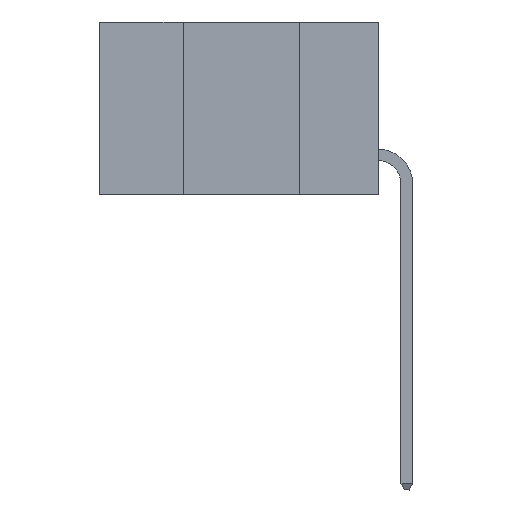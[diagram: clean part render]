
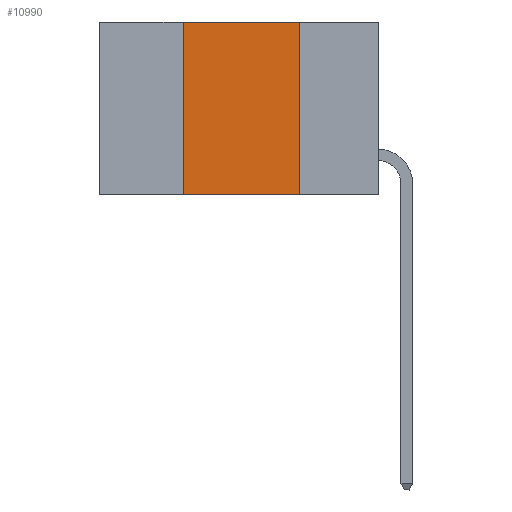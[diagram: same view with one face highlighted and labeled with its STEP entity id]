
A CAD part, left-side view. The second image highlights one B-rep face of the part: STEP entity #10990.
In plain terms, the highlighted planar face has unit normal (-1, 0, 0).
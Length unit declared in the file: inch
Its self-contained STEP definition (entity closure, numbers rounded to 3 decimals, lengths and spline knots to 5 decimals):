
#491 = EDGE_CURVE ( 'NONE', #5956, #13332, #5429, .T. ) ;
#874 = EDGE_LOOP ( 'NONE', ( #14414, #11052, #2569, #13044 ) ) ;
#1009 = DIRECTION ( 'NONE',  ( 0., 0., 1. ) ) ;
#1299 = DIRECTION ( 'NONE',  ( 0., -1., 0. ) ) ;
#2569 = ORIENTED_EDGE ( 'NONE', *, *, #491, .F. ) ;
#2683 = CARTESIAN_POINT ( 'NONE',  ( 0., 0.6, 0. ) ) ;
#2935 = VERTEX_POINT ( 'NONE', #14558 ) ;
#2951 = CARTESIAN_POINT ( 'NONE',  ( 0., 0.42, 0. ) ) ;
#3145 = EDGE_CURVE ( 'NONE', #2935, #16060, #17290, .T. ) ;
#4485 = PLANE ( 'NONE',  #13430 ) ;
#5429 = LINE ( 'NONE', #13811, #9124 ) ;
#5556 = LINE ( 'NONE', #15498, #8524 ) ;
#5648 = EDGE_CURVE ( 'NONE', #13332, #2935, #5556, .T. ) ;
#5956 = VERTEX_POINT ( 'NONE', #14962 ) ;
#7456 = CARTESIAN_POINT ( 'NONE',  ( 0., 0.17, -0.37 ) ) ;
#7720 = DIRECTION ( 'NONE',  ( 0., -1., 0. ) ) ;
#8524 = VECTOR ( 'NONE', #1299, 39.37008 ) ;
#8714 = FACE_OUTER_BOUND ( 'NONE', #874, .T. ) ;
#9124 = VECTOR ( 'NONE', #1009, 39.37008 ) ;
#9308 = VECTOR ( 'NONE', #7720, 39.37008 ) ;
#10055 = VECTOR ( 'NONE', #11528, 39.37008 ) ;
#10190 = LINE ( 'NONE', #11851, #9308 ) ;
#10990 = ADVANCED_FACE ( 'NONE', ( #8714 ), #4485, .F. ) ;
#11052 = ORIENTED_EDGE ( 'NONE', *, *, #5648, .F. ) ;
#11528 = DIRECTION ( 'NONE',  ( 0., 0., -1. ) ) ;
#11851 = CARTESIAN_POINT ( 'NONE',  ( 0., 0.6, -0.37 ) ) ;
#13044 = ORIENTED_EDGE ( 'NONE', *, *, #17074, .T. ) ;
#13332 = VERTEX_POINT ( 'NONE', #2951 ) ;
#13430 = AXIS2_PLACEMENT_3D ( 'NONE', #2683, #14338, #15842 ) ;
#13811 = CARTESIAN_POINT ( 'NONE',  ( 0., 0.42, -0.37 ) ) ;
#14338 = DIRECTION ( 'NONE',  ( 1., 0., 0. ) ) ;
#14414 = ORIENTED_EDGE ( 'NONE', *, *, #3145, .F. ) ;
#14558 = CARTESIAN_POINT ( 'NONE',  ( 0., 0.17, 0. ) ) ;
#14962 = CARTESIAN_POINT ( 'NONE',  ( 0., 0.42, -0.37 ) ) ;
#15498 = CARTESIAN_POINT ( 'NONE',  ( 0., 0.6, 0. ) ) ;
#15842 = DIRECTION ( 'NONE',  ( 0., 0., -1. ) ) ;
#16060 = VERTEX_POINT ( 'NONE', #17457 ) ;
#17074 = EDGE_CURVE ( 'NONE', #5956, #16060, #10190, .T. ) ;
#17290 = LINE ( 'NONE', #7456, #10055 ) ;
#17457 = CARTESIAN_POINT ( 'NONE',  ( 0., 0.17, -0.37 ) ) ;
